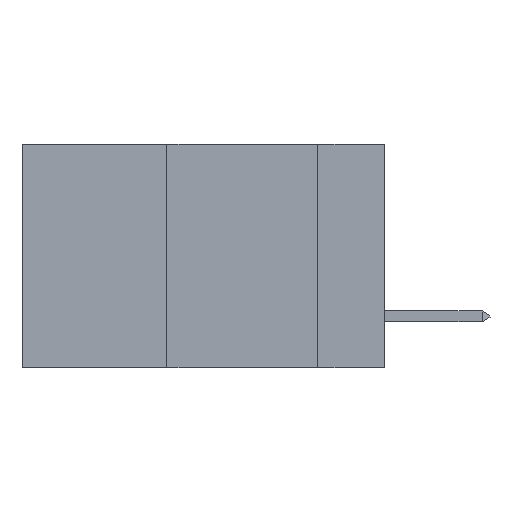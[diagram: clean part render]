
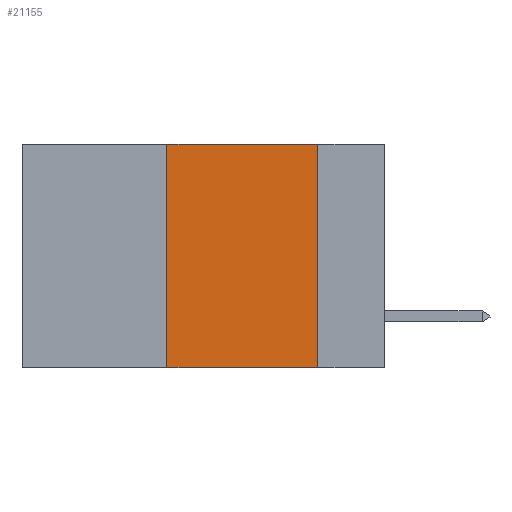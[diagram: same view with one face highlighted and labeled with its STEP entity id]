
A CAD part, left-side view. The second image highlights one B-rep face of the part: STEP entity #21155.
In plain terms, the highlighted planar face has unit normal (-1, 0, 0).
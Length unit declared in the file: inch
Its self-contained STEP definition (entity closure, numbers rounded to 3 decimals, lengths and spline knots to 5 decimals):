
#2911 = ORIENTED_EDGE ( 'NONE', *, *, #18489, .F. ) ;
#4217 = EDGE_CURVE ( 'NONE', #11918, #11676, #28938, .T. ) ;
#4410 = ORIENTED_EDGE ( 'NONE', *, *, #14493, .F. ) ;
#4610 = VECTOR ( 'NONE', #4839, 39.37008 ) ;
#4636 = DIRECTION ( 'NONE',  ( 0., -1., 0. ) ) ;
#4839 = DIRECTION ( 'NONE',  ( 0., -1., 0. ) ) ;
#5339 = CARTESIAN_POINT ( 'NONE',  ( 0., 0.6, 0. ) ) ;
#6080 = VECTOR ( 'NONE', #12257, 39.37008 ) ;
#7708 = DIRECTION ( 'NONE',  ( 0., 0., -1. ) ) ;
#9304 = DIRECTION ( 'NONE',  ( 0., 0., -1. ) ) ;
#9370 = CARTESIAN_POINT ( 'NONE',  ( 0., 0.6, 0. ) ) ;
#10538 = EDGE_CURVE ( 'NONE', #11918, #18915, #18663, .T. ) ;
#11676 = VERTEX_POINT ( 'NONE', #14185 ) ;
#11918 = VERTEX_POINT ( 'NONE', #24332 ) ;
#12257 = DIRECTION ( 'NONE',  ( 0., 0., 1. ) ) ;
#13549 = CARTESIAN_POINT ( 'NONE',  ( 0., 0.11, 0. ) ) ;
#13828 = VECTOR ( 'NONE', #9304, 39.37008 ) ;
#14009 = FACE_OUTER_BOUND ( 'NONE', #17774, .T. ) ;
#14185 = CARTESIAN_POINT ( 'NONE',  ( 0., 0.11, -0.37 ) ) ;
#14493 = EDGE_CURVE ( 'NONE', #18915, #20784, #17828, .T. ) ;
#16481 = CARTESIAN_POINT ( 'NONE',  ( 0., 0.11, 0. ) ) ;
#17774 = EDGE_LOOP ( 'NONE', ( #2911, #4410, #25042, #26637 ) ) ;
#17828 = LINE ( 'NONE', #9370, #30263 ) ;
#18489 = EDGE_CURVE ( 'NONE', #20784, #11676, #30344, .T. ) ;
#18663 = LINE ( 'NONE', #21650, #6080 ) ;
#18915 = VERTEX_POINT ( 'NONE', #22590 ) ;
#19008 = CARTESIAN_POINT ( 'NONE',  ( 0., 0.6, -0.37 ) ) ;
#20784 = VERTEX_POINT ( 'NONE', #13549 ) ;
#21155 = ADVANCED_FACE ( 'NONE', ( #14009 ), #28828, .F. ) ;
#21650 = CARTESIAN_POINT ( 'NONE',  ( 0., 0.36, 0. ) ) ;
#21856 = DIRECTION ( 'NONE',  ( 1., 0., 0. ) ) ;
#22590 = CARTESIAN_POINT ( 'NONE',  ( 0., 0.36, 0. ) ) ;
#24332 = CARTESIAN_POINT ( 'NONE',  ( 0., 0.36, -0.37 ) ) ;
#25042 = ORIENTED_EDGE ( 'NONE', *, *, #10538, .F. ) ;
#26637 = ORIENTED_EDGE ( 'NONE', *, *, #4217, .T. ) ;
#28828 = PLANE ( 'NONE',  #30628 ) ;
#28938 = LINE ( 'NONE', #19008, #4610 ) ;
#30263 = VECTOR ( 'NONE', #4636, 39.37008 ) ;
#30344 = LINE ( 'NONE', #16481, #13828 ) ;
#30628 = AXIS2_PLACEMENT_3D ( 'NONE', #5339, #21856, #7708 ) ;
